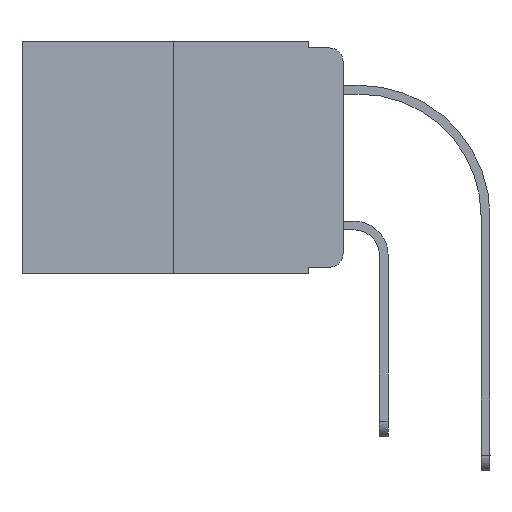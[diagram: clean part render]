
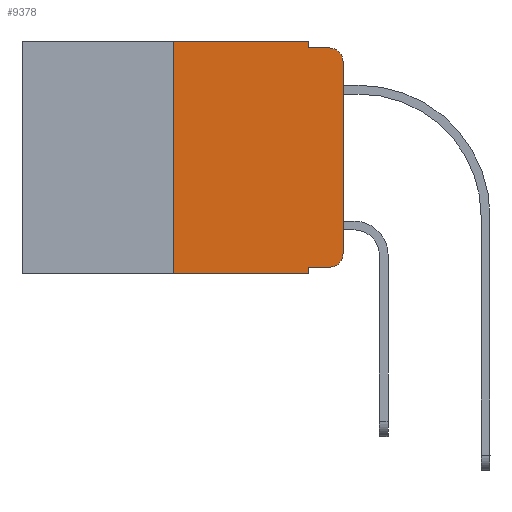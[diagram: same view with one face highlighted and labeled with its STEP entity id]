
A CAD part, left-side view. The second image highlights one B-rep face of the part: STEP entity #9378.
In plain terms, the highlighted planar face has unit normal (-1, 0, 0).
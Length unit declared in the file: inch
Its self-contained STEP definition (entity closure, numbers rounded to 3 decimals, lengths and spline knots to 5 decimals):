
#122 = DIRECTION ( 'NONE',  ( 0., 0., -1. ) ) ;
#138 = EDGE_CURVE ( 'NONE', #4356, #13705, #10775, .T. ) ;
#194 = DIRECTION ( 'NONE',  ( 0., 0., -1. ) ) ;
#452 = VERTEX_POINT ( 'NONE', #2178 ) ;
#553 = DIRECTION ( 'NONE',  ( 0., -1., 0. ) ) ;
#692 = CARTESIAN_POINT ( 'NONE',  ( 0., 0.051, -0.343 ) ) ;
#1018 = DIRECTION ( 'NONE',  ( 0., -1., 0. ) ) ;
#1051 = EDGE_CURVE ( 'NONE', #452, #2660, #3715, .T. ) ;
#1059 = ORIENTED_EDGE ( 'NONE', *, *, #7542, .T. ) ;
#2033 = VECTOR ( 'NONE', #4063, 39.37008 ) ;
#2117 = VECTOR ( 'NONE', #553, 39.37008 ) ;
#2178 = CARTESIAN_POINT ( 'NONE',  ( 0., 0.051, -0.333 ) ) ;
#2218 = ORIENTED_EDGE ( 'NONE', *, *, #138, .F. ) ;
#2451 = DIRECTION ( 'NONE',  ( -1., 0., 0. ) ) ;
#2453 = LINE ( 'NONE', #5957, #12638 ) ;
#2623 = VECTOR ( 'NONE', #122, 39.37008 ) ;
#2642 = VERTEX_POINT ( 'NONE', #692 ) ;
#2659 = DIRECTION ( 'NONE',  ( 0., 0., -1. ) ) ;
#2660 = VERTEX_POINT ( 'NONE', #8872 ) ;
#2826 = CARTESIAN_POINT ( 'NONE',  ( 0., 0.25, -0.343 ) ) ;
#3110 = ORIENTED_EDGE ( 'NONE', *, *, #11600, .T. ) ;
#3139 = CARTESIAN_POINT ( 'NONE',  ( 0., 0.051, 0. ) ) ;
#3217 = AXIS2_PLACEMENT_3D ( 'NONE', #4380, #2451, #9242 ) ;
#3306 = ORIENTED_EDGE ( 'NONE', *, *, #11943, .F. ) ;
#3351 = DIRECTION ( 'NONE',  ( 0., 0., -1. ) ) ;
#3458 = AXIS2_PLACEMENT_3D ( 'NONE', #8139, #13589, #3351 ) ;
#3715 = LINE ( 'NONE', #12848, #2117 ) ;
#3788 = ORIENTED_EDGE ( 'NONE', *, *, #8308, .T. ) ;
#3802 = VERTEX_POINT ( 'NONE', #12312 ) ;
#4063 = DIRECTION ( 'NONE',  ( 0., -1., 0. ) ) ;
#4082 = VERTEX_POINT ( 'NONE', #12925 ) ;
#4356 = VERTEX_POINT ( 'NONE', #2826 ) ;
#4380 = CARTESIAN_POINT ( 'NONE',  ( 0., 0.02, -0.03 ) ) ;
#4465 = PLANE ( 'NONE',  #3458 ) ;
#5073 = ORIENTED_EDGE ( 'NONE', *, *, #13992, .F. ) ;
#5199 = DIRECTION ( 'NONE',  ( 0., -1., 0. ) ) ;
#5248 = ORIENTED_EDGE ( 'NONE', *, *, #1051, .T. ) ;
#5763 = LINE ( 'NONE', #6664, #6617 ) ;
#5808 = VERTEX_POINT ( 'NONE', #3139 ) ;
#5957 = CARTESIAN_POINT ( 'NONE',  ( 0., 0., 0. ) ) ;
#6617 = VECTOR ( 'NONE', #1018, 39.37008 ) ;
#6664 = CARTESIAN_POINT ( 'NONE',  ( 0., 0.473, 0. ) ) ;
#7542 = EDGE_CURVE ( 'NONE', #10347, #9697, #13005, .T. ) ;
#7673 = CARTESIAN_POINT ( 'NONE',  ( 0., 0.02, -0.01 ) ) ;
#7716 = VECTOR ( 'NONE', #194, 39.37008 ) ;
#7729 = CARTESIAN_POINT ( 'NONE',  ( 0., 0.051, -0.01 ) ) ;
#8139 = CARTESIAN_POINT ( 'NONE',  ( 0., 0.473, 0. ) ) ;
#8294 = LINE ( 'NONE', #10370, #7716 ) ;
#8308 = EDGE_CURVE ( 'NONE', #4356, #2642, #8555, .T. ) ;
#8555 = LINE ( 'NONE', #11975, #2033 ) ;
#8872 = CARTESIAN_POINT ( 'NONE',  ( 0., 0.02, -0.333 ) ) ;
#9211 = ORIENTED_EDGE ( 'NONE', *, *, #11326, .F. ) ;
#9242 = DIRECTION ( 'NONE',  ( 0., 0., -1. ) ) ;
#9378 = ADVANCED_FACE ( 'NONE', ( #11631 ), #4465, .F. ) ;
#9550 = DIRECTION ( 'NONE',  ( 0., 0., 1. ) ) ;
#9697 = VERTEX_POINT ( 'NONE', #7673 ) ;
#9717 = CARTESIAN_POINT ( 'NONE',  ( 0., 0., -0.03 ) ) ;
#9949 = CIRCLE ( 'NONE', #14727, 0.02 ) ;
#10305 = CARTESIAN_POINT ( 'NONE',  ( 0., 0.051, 0. ) ) ;
#10347 = VERTEX_POINT ( 'NONE', #9717 ) ;
#10370 = CARTESIAN_POINT ( 'NONE',  ( 0., 0.051, 0. ) ) ;
#10775 = LINE ( 'NONE', #14072, #12326 ) ;
#10981 = DIRECTION ( 'NONE',  ( -1., 0., 0. ) ) ;
#11326 = EDGE_CURVE ( 'NONE', #4082, #9697, #13338, .T. ) ;
#11421 = LINE ( 'NONE', #10305, #2623 ) ;
#11600 = EDGE_CURVE ( 'NONE', #2660, #3802, #9949, .T. ) ;
#11631 = FACE_OUTER_BOUND ( 'NONE', #12946, .T. ) ;
#11740 = DIRECTION ( 'NONE',  ( 0., 0., 1. ) ) ;
#11749 = CARTESIAN_POINT ( 'NONE',  ( 0., 0.02, -0.313 ) ) ;
#11943 = EDGE_CURVE ( 'NONE', #452, #2642, #8294, .T. ) ;
#11975 = CARTESIAN_POINT ( 'NONE',  ( 0., 0.473, -0.343 ) ) ;
#12262 = EDGE_CURVE ( 'NONE', #13705, #5808, #5763, .T. ) ;
#12312 = CARTESIAN_POINT ( 'NONE',  ( 0., 0., -0.313 ) ) ;
#12326 = VECTOR ( 'NONE', #11740, 39.37008 ) ;
#12638 = VECTOR ( 'NONE', #9550, 39.37008 ) ;
#12848 = CARTESIAN_POINT ( 'NONE',  ( 0., 0.051, -0.333 ) ) ;
#12863 = ORIENTED_EDGE ( 'NONE', *, *, #12262, .F. ) ;
#12919 = ORIENTED_EDGE ( 'NONE', *, *, #14450, .T. ) ;
#12925 = CARTESIAN_POINT ( 'NONE',  ( 0., 0.051, -0.01 ) ) ;
#12946 = EDGE_LOOP ( 'NONE', ( #12919, #1059, #9211, #5073, #12863, #2218, #3788, #3306, #5248, #3110 ) ) ;
#13005 = CIRCLE ( 'NONE', #3217, 0.02 ) ;
#13093 = CARTESIAN_POINT ( 'NONE',  ( 0., 0.25, 0. ) ) ;
#13338 = LINE ( 'NONE', #7729, #14249 ) ;
#13589 = DIRECTION ( 'NONE',  ( 1., 0., 0. ) ) ;
#13705 = VERTEX_POINT ( 'NONE', #13093 ) ;
#13992 = EDGE_CURVE ( 'NONE', #5808, #4082, #11421, .T. ) ;
#14072 = CARTESIAN_POINT ( 'NONE',  ( 0., 0.25, 0. ) ) ;
#14249 = VECTOR ( 'NONE', #5199, 39.37008 ) ;
#14450 = EDGE_CURVE ( 'NONE', #3802, #10347, #2453, .T. ) ;
#14727 = AXIS2_PLACEMENT_3D ( 'NONE', #11749, #10981, #2659 ) ;
